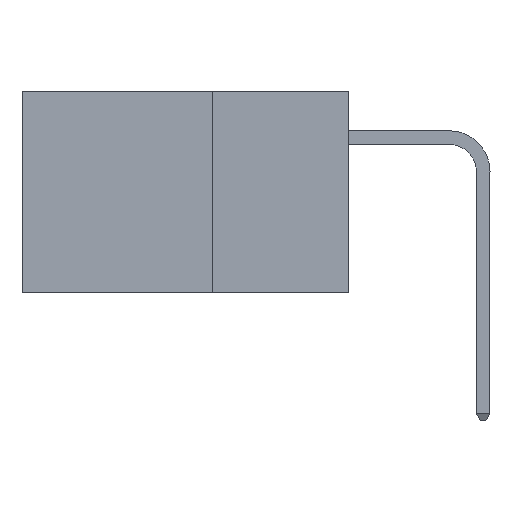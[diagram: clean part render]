
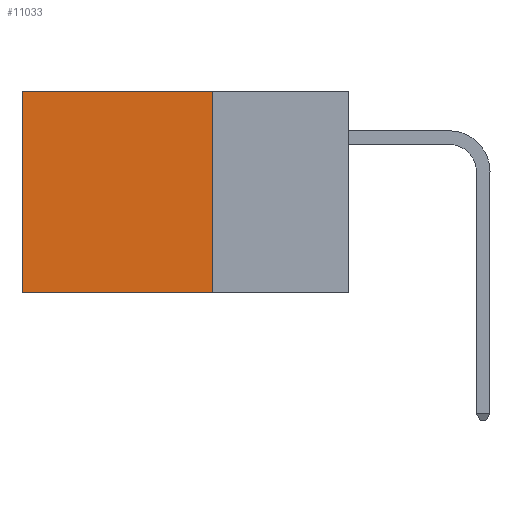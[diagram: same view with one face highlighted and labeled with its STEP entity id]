
A CAD part, left-side view. The second image highlights one B-rep face of the part: STEP entity #11033.
In plain terms, the highlighted planar face has unit normal (-1, 0, 0).
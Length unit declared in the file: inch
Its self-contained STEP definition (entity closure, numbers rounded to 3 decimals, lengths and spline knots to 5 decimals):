
#1279 = CARTESIAN_POINT ( 'NONE',  ( 0.2875, 0.25, 0. ) ) ;
#2241 = ORIENTED_EDGE ( 'NONE', *, *, #29419, .T. ) ;
#4816 = EDGE_CURVE ( 'NONE', #23546, #29659, #36649, .T. ) ;
#5701 = DIRECTION ( 'NONE',  ( 0., 1., 0. ) ) ;
#5721 = PLANE ( 'NONE',  #6182 ) ;
#6085 = VECTOR ( 'NONE', #17777, 39.37008 ) ;
#6182 = AXIS2_PLACEMENT_3D ( 'NONE', #28724, #11540, #28848 ) ;
#8158 = LINE ( 'NONE', #11519, #14000 ) ;
#8531 = LINE ( 'NONE', #36336, #24273 ) ;
#9160 = CARTESIAN_POINT ( 'NONE',  ( 0.2875, 0.6, -0.37 ) ) ;
#9435 = ORIENTED_EDGE ( 'NONE', *, *, #32793, .T. ) ;
#11033 = ADVANCED_FACE ( 'NONE', ( #18211 ), #5721, .F. ) ;
#11519 = CARTESIAN_POINT ( 'NONE',  ( 0.2875, 0.25, -0.37 ) ) ;
#11540 = DIRECTION ( 'NONE',  ( 1., 0., 0. ) ) ;
#14000 = VECTOR ( 'NONE', #5701, 39.37008 ) ;
#15388 = DIRECTION ( 'NONE',  ( 0., 1., 0. ) ) ;
#16743 = CARTESIAN_POINT ( 'NONE',  ( 0.2875, 0.25, -0.37 ) ) ;
#17751 = CARTESIAN_POINT ( 'NONE',  ( 0.2875, 0.6, 0. ) ) ;
#17777 = DIRECTION ( 'NONE',  ( 0., 0., -1. ) ) ;
#17789 = VECTOR ( 'NONE', #15388, 39.37008 ) ;
#17961 = EDGE_LOOP ( 'NONE', ( #9435, #23172, #34629, #2241 ) ) ;
#18211 = FACE_OUTER_BOUND ( 'NONE', #17961, .T. ) ;
#19166 = EDGE_CURVE ( 'NONE', #29659, #33809, #8158, .T. ) ;
#23172 = ORIENTED_EDGE ( 'NONE', *, *, #19166, .F. ) ;
#23537 = CARTESIAN_POINT ( 'NONE',  ( 0.2875, 0.25, 0. ) ) ;
#23546 = VERTEX_POINT ( 'NONE', #28341 ) ;
#24273 = VECTOR ( 'NONE', #33211, 39.37008 ) ;
#28341 = CARTESIAN_POINT ( 'NONE',  ( 0.2875, 0.25, 0. ) ) ;
#28535 = LINE ( 'NONE', #1279, #17789 ) ;
#28724 = CARTESIAN_POINT ( 'NONE',  ( 0.2875, 0.25, 0. ) ) ;
#28848 = DIRECTION ( 'NONE',  ( 0., 0., -1. ) ) ;
#29419 = EDGE_CURVE ( 'NONE', #23546, #33181, #28535, .T. ) ;
#29659 = VERTEX_POINT ( 'NONE', #16743 ) ;
#32793 = EDGE_CURVE ( 'NONE', #33181, #33809, #8531, .T. ) ;
#33181 = VERTEX_POINT ( 'NONE', #17751 ) ;
#33211 = DIRECTION ( 'NONE',  ( 0., 0., -1. ) ) ;
#33809 = VERTEX_POINT ( 'NONE', #9160 ) ;
#34629 = ORIENTED_EDGE ( 'NONE', *, *, #4816, .F. ) ;
#36336 = CARTESIAN_POINT ( 'NONE',  ( 0.2875, 0.6, 0. ) ) ;
#36649 = LINE ( 'NONE', #23537, #6085 ) ;
